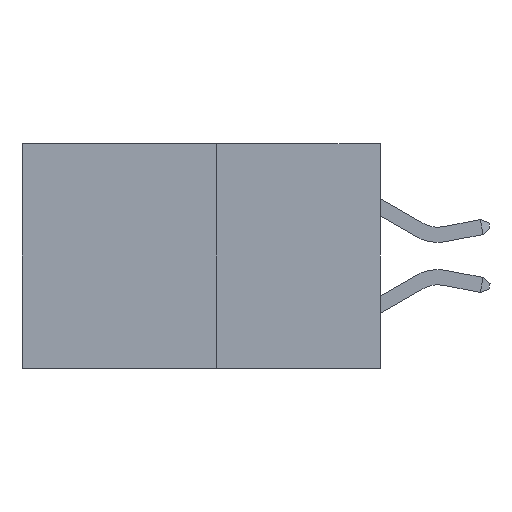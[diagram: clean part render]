
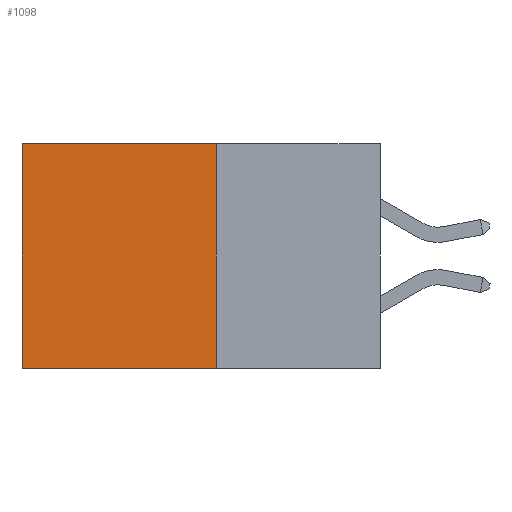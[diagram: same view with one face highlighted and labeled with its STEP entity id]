
A CAD part, left-side view. The second image highlights one B-rep face of the part: STEP entity #1098.
In plain terms, the highlighted planar face has unit normal (-1, 0, 0).
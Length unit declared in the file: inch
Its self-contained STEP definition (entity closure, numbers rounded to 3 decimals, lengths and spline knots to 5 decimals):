
#619 = VERTEX_POINT ( 'NONE', #3302 ) ;
#677 = ORIENTED_EDGE ( 'NONE', *, *, #2013, .F. ) ;
#806 = ORIENTED_EDGE ( 'NONE', *, *, #2050, .T. ) ;
#1098 = ADVANCED_FACE ( 'NONE', ( #7092 ), #8152, .F. ) ;
#1384 = EDGE_CURVE ( 'NONE', #619, #1900, #6555, .T. ) ;
#1671 = VECTOR ( 'NONE', #3055, 39.37008 ) ;
#1900 = VERTEX_POINT ( 'NONE', #6741 ) ;
#2013 = EDGE_CURVE ( 'NONE', #1900, #3096, #8578, .T. ) ;
#2050 = EDGE_CURVE ( 'NONE', #5295, #3096, #7076, .T. ) ;
#2912 = AXIS2_PLACEMENT_3D ( 'NONE', #8119, #7408, #6465 ) ;
#2962 = VECTOR ( 'NONE', #4965, 39.37008 ) ;
#3055 = DIRECTION ( 'NONE',  ( 0., 1., 0. ) ) ;
#3096 = VERTEX_POINT ( 'NONE', #4729 ) ;
#3177 = DIRECTION ( 'NONE',  ( 0., 1., 0. ) ) ;
#3302 = CARTESIAN_POINT ( 'NONE',  ( 0.277, 0.27, 0. ) ) ;
#3696 = CARTESIAN_POINT ( 'NONE',  ( 0.277, 0.27, -0.37 ) ) ;
#4412 = CARTESIAN_POINT ( 'NONE',  ( 0.277, 0.59, 0. ) ) ;
#4729 = CARTESIAN_POINT ( 'NONE',  ( 0.277, 0.59, -0.37 ) ) ;
#4965 = DIRECTION ( 'NONE',  ( 0., 0., -1. ) ) ;
#5048 = CARTESIAN_POINT ( 'NONE',  ( 0.277, 0.59, -0.37 ) ) ;
#5066 = EDGE_CURVE ( 'NONE', #619, #5295, #6402, .T. ) ;
#5295 = VERTEX_POINT ( 'NONE', #4412 ) ;
#5523 = CARTESIAN_POINT ( 'NONE',  ( 0.277, 0.27, -0.37 ) ) ;
#6071 = ORIENTED_EDGE ( 'NONE', *, *, #1384, .F. ) ;
#6385 = ORIENTED_EDGE ( 'NONE', *, *, #5066, .T. ) ;
#6402 = LINE ( 'NONE', #7660, #8160 ) ;
#6465 = DIRECTION ( 'NONE',  ( 0., 0., -1. ) ) ;
#6555 = LINE ( 'NONE', #5523, #2962 ) ;
#6741 = CARTESIAN_POINT ( 'NONE',  ( 0.277, 0.27, -0.37 ) ) ;
#7076 = LINE ( 'NONE', #5048, #8388 ) ;
#7092 = FACE_OUTER_BOUND ( 'NONE', #7887, .T. ) ;
#7282 = DIRECTION ( 'NONE',  ( 0., 0., -1. ) ) ;
#7408 = DIRECTION ( 'NONE',  ( 1., 0., 0. ) ) ;
#7660 = CARTESIAN_POINT ( 'NONE',  ( 0.277, 0.27, 0. ) ) ;
#7887 = EDGE_LOOP ( 'NONE', ( #806, #677, #6071, #6385 ) ) ;
#8119 = CARTESIAN_POINT ( 'NONE',  ( 0.277, 0.27, -0.37 ) ) ;
#8152 = PLANE ( 'NONE',  #2912 ) ;
#8160 = VECTOR ( 'NONE', #3177, 39.37008 ) ;
#8388 = VECTOR ( 'NONE', #7282, 39.37008 ) ;
#8578 = LINE ( 'NONE', #3696, #1671 ) ;
